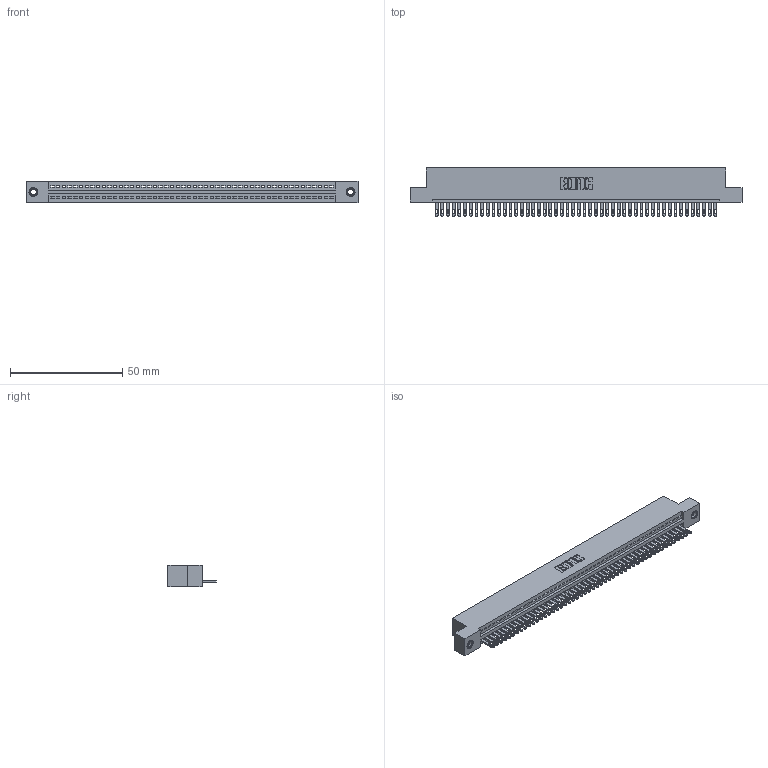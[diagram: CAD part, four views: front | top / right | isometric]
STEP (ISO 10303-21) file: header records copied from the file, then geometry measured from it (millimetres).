
FILE_DESCRIPTION (( 'STEP AP203' ), '1' );
FILE_NAME ('895-050-500-107.STEP', '2020-09-27T08:40:30', ( '' ), ( '' ), 'SwSTEP 2.0', 'SolidWorks 2020', '' );
FILE_SCHEMA (( 'CONFIG_CONTROL_DESIGN' ));
Length unit declared in the file: inch
Products named in the file (4): 895-050-500-107; 345-250-001_345-250-005-103; 845 Part_Flush Mounting Lugs - 0.156 Dia-TI; 345-292-001_345-293-100
Assembly tree (53 placements, depth 2):
  895-050-500-107
    845 Part_Flush Mounting Lugs - 0.156 Dia-TI
    345-292-001_345-293-100  x50
    345-250-001_345-250-005-103  x2
Bounding box: 148.21 x 21.51 x 9.4 mm (x, y, z)
Volume: 14160 mm3; surface area: 19070.9 mm2
Topology: 53 solids, 53 shells, 2886 faces, 8877 edges, 5910 vertices
Faces by surface type: plane 1812, cylinder 1058, cone 12, torus 4
Entity records: 37670 total; most frequent: CARTESIAN_POINT 6505, ORIENTED_EDGE 6482, DIRECTION 5699, EDGE_CURVE 3241, VECTOR 2885, LINE 2885, VERTEX_POINT 2156, AXIS2_PLACEMENT_3D 1407
